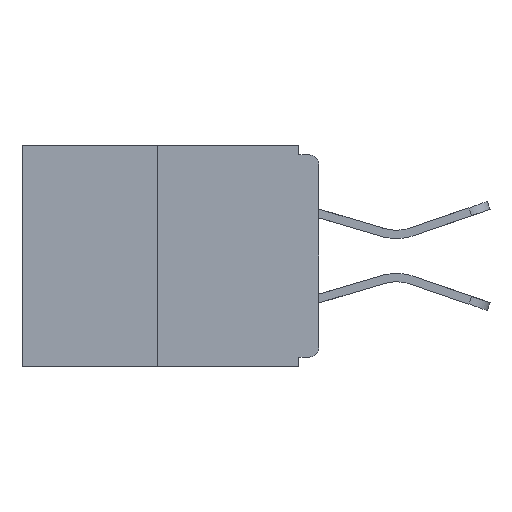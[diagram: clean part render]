
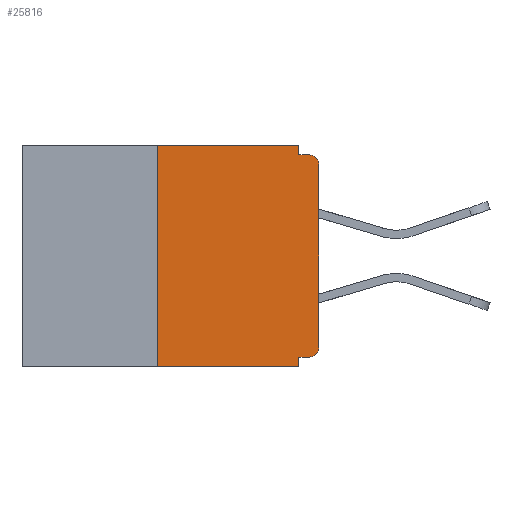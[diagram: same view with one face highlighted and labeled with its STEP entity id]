
A CAD part, left-side view. The second image highlights one B-rep face of the part: STEP entity #25816.
In plain terms, the highlighted planar face has unit normal (-1, 0, 0).
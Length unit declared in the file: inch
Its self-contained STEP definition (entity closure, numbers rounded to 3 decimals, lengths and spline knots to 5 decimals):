
#410 = CARTESIAN_POINT ( 'NONE',  ( 0., 0.015, -0.313 ) ) ;
#488 = CARTESIAN_POINT ( 'NONE',  ( 0., 0.46, 0. ) ) ;
#631 = DIRECTION ( 'NONE',  ( 0., 0., -1. ) ) ;
#680 = VERTEX_POINT ( 'NONE', #16610 ) ;
#861 = EDGE_CURVE ( 'NONE', #23442, #680, #24051, .T. ) ;
#1447 = VERTEX_POINT ( 'NONE', #28276 ) ;
#2391 = ORIENTED_EDGE ( 'NONE', *, *, #11035, .F. ) ;
#2514 = CARTESIAN_POINT ( 'NONE',  ( 0., 0.031, 0. ) ) ;
#2586 = VERTEX_POINT ( 'NONE', #2514 ) ;
#3082 = VERTEX_POINT ( 'NONE', #15944 ) ;
#3655 = VECTOR ( 'NONE', #28322, 39.37008 ) ;
#3971 = EDGE_CURVE ( 'NONE', #19951, #1447, #17359, .T. ) ;
#4835 = DIRECTION ( 'NONE',  ( 0., 0., 1. ) ) ;
#4918 = ORIENTED_EDGE ( 'NONE', *, *, #15666, .F. ) ;
#5363 = FACE_OUTER_BOUND ( 'NONE', #6683, .T. ) ;
#5620 = AXIS2_PLACEMENT_3D ( 'NONE', #19392, #25793, #17046 ) ;
#6114 = DIRECTION ( 'NONE',  ( 0., -1., 0. ) ) ;
#6511 = CARTESIAN_POINT ( 'NONE',  ( 0., 0.25, 0. ) ) ;
#6683 = EDGE_LOOP ( 'NONE', ( #23145, #2391, #7792, #4918, #27323, #22027, #7828, #22195, #7164, #7890 ) ) ;
#7164 = ORIENTED_EDGE ( 'NONE', *, *, #12811, .F. ) ;
#7316 = VECTOR ( 'NONE', #8684, 39.37008 ) ;
#7741 = DIRECTION ( 'NONE',  ( 0., 0., 1. ) ) ;
#7792 = ORIENTED_EDGE ( 'NONE', *, *, #3971, .T. ) ;
#7828 = ORIENTED_EDGE ( 'NONE', *, *, #26403, .T. ) ;
#7890 = ORIENTED_EDGE ( 'NONE', *, *, #22466, .F. ) ;
#8588 = LINE ( 'NONE', #17633, #3655 ) ;
#8684 = DIRECTION ( 'NONE',  ( 0., 0., -1. ) ) ;
#8834 = EDGE_CURVE ( 'NONE', #13036, #2586, #26666, .T. ) ;
#8872 = CARTESIAN_POINT ( 'NONE',  ( 0., 0.031, -0.328 ) ) ;
#10228 = LINE ( 'NONE', #12006, #11800 ) ;
#10923 = CARTESIAN_POINT ( 'NONE',  ( 0., 0.031, -0.343 ) ) ;
#11035 = EDGE_CURVE ( 'NONE', #19951, #13036, #19556, .T. ) ;
#11478 = CARTESIAN_POINT ( 'NONE',  ( 0., 0.015, -0.328 ) ) ;
#11800 = VECTOR ( 'NONE', #19234, 39.37008 ) ;
#11997 = VERTEX_POINT ( 'NONE', #28533 ) ;
#12006 = CARTESIAN_POINT ( 'NONE',  ( 0., 0., -0.015 ) ) ;
#12811 = EDGE_CURVE ( 'NONE', #11997, #680, #10228, .T. ) ;
#13036 = VERTEX_POINT ( 'NONE', #6511 ) ;
#13260 = AXIS2_PLACEMENT_3D ( 'NONE', #488, #21315, #631 ) ;
#13624 = VERTEX_POINT ( 'NONE', #8872 ) ;
#14301 = LINE ( 'NONE', #16230, #22252 ) ;
#14853 = VECTOR ( 'NONE', #22217, 39.37008 ) ;
#14879 = CIRCLE ( 'NONE', #15361, 0.015 ) ;
#15361 = AXIS2_PLACEMENT_3D ( 'NONE', #410, #18442, #23177 ) ;
#15666 = EDGE_CURVE ( 'NONE', #13624, #1447, #24654, .T. ) ;
#15944 = CARTESIAN_POINT ( 'NONE',  ( 0., 0., -0.313 ) ) ;
#16230 = CARTESIAN_POINT ( 'NONE',  ( 0., 0., 0. ) ) ;
#16610 = CARTESIAN_POINT ( 'NONE',  ( 0., 0.015, -0.015 ) ) ;
#17046 = DIRECTION ( 'NONE',  ( 0., 0., -1. ) ) ;
#17207 = EDGE_CURVE ( 'NONE', #19925, #3082, #14879, .T. ) ;
#17359 = LINE ( 'NONE', #26378, #23916 ) ;
#17633 = CARTESIAN_POINT ( 'NONE',  ( 0., 0.031, 0. ) ) ;
#17789 = CARTESIAN_POINT ( 'NONE',  ( 0., 0.46, 0. ) ) ;
#18442 = DIRECTION ( 'NONE',  ( -1., 0., 0. ) ) ;
#18869 = VECTOR ( 'NONE', #7741, 39.37008 ) ;
#19022 = VECTOR ( 'NONE', #27560, 39.37008 ) ;
#19234 = DIRECTION ( 'NONE',  ( 0., -1., 0. ) ) ;
#19392 = CARTESIAN_POINT ( 'NONE',  ( 0., 0.015, -0.03 ) ) ;
#19556 = LINE ( 'NONE', #25954, #18869 ) ;
#19925 = VERTEX_POINT ( 'NONE', #11478 ) ;
#19951 = VERTEX_POINT ( 'NONE', #29123 ) ;
#21315 = DIRECTION ( 'NONE',  ( 1., 0., 0. ) ) ;
#22027 = ORIENTED_EDGE ( 'NONE', *, *, #17207, .T. ) ;
#22195 = ORIENTED_EDGE ( 'NONE', *, *, #861, .T. ) ;
#22217 = DIRECTION ( 'NONE',  ( 0., -1., 0. ) ) ;
#22252 = VECTOR ( 'NONE', #4835, 39.37008 ) ;
#22466 = EDGE_CURVE ( 'NONE', #2586, #11997, #8588, .T. ) ;
#23145 = ORIENTED_EDGE ( 'NONE', *, *, #8834, .F. ) ;
#23177 = DIRECTION ( 'NONE',  ( 0., 0., -1. ) ) ;
#23415 = PLANE ( 'NONE',  #13260 ) ;
#23442 = VERTEX_POINT ( 'NONE', #28831 ) ;
#23916 = VECTOR ( 'NONE', #6114, 39.37008 ) ;
#24051 = CIRCLE ( 'NONE', #5620, 0.015 ) ;
#24654 = LINE ( 'NONE', #10923, #7316 ) ;
#25044 = LINE ( 'NONE', #28277, #19022 ) ;
#25793 = DIRECTION ( 'NONE',  ( -1., 0., 0. ) ) ;
#25816 = ADVANCED_FACE ( 'NONE', ( #5363 ), #23415, .F. ) ;
#25954 = CARTESIAN_POINT ( 'NONE',  ( 0., 0.25, 0. ) ) ;
#26378 = CARTESIAN_POINT ( 'NONE',  ( 0., 0.46, -0.343 ) ) ;
#26403 = EDGE_CURVE ( 'NONE', #3082, #23442, #14301, .T. ) ;
#26666 = LINE ( 'NONE', #17789, #14853 ) ;
#27323 = ORIENTED_EDGE ( 'NONE', *, *, #28637, .F. ) ;
#27560 = DIRECTION ( 'NONE',  ( 0., 1., 0. ) ) ;
#28276 = CARTESIAN_POINT ( 'NONE',  ( 0., 0.031, -0.343 ) ) ;
#28277 = CARTESIAN_POINT ( 'NONE',  ( 0., 0., -0.328 ) ) ;
#28322 = DIRECTION ( 'NONE',  ( 0., 0., -1. ) ) ;
#28533 = CARTESIAN_POINT ( 'NONE',  ( 0., 0.031, -0.015 ) ) ;
#28637 = EDGE_CURVE ( 'NONE', #19925, #13624, #25044, .T. ) ;
#28831 = CARTESIAN_POINT ( 'NONE',  ( 0., 0., -0.03 ) ) ;
#29123 = CARTESIAN_POINT ( 'NONE',  ( 0., 0.25, -0.343 ) ) ;
